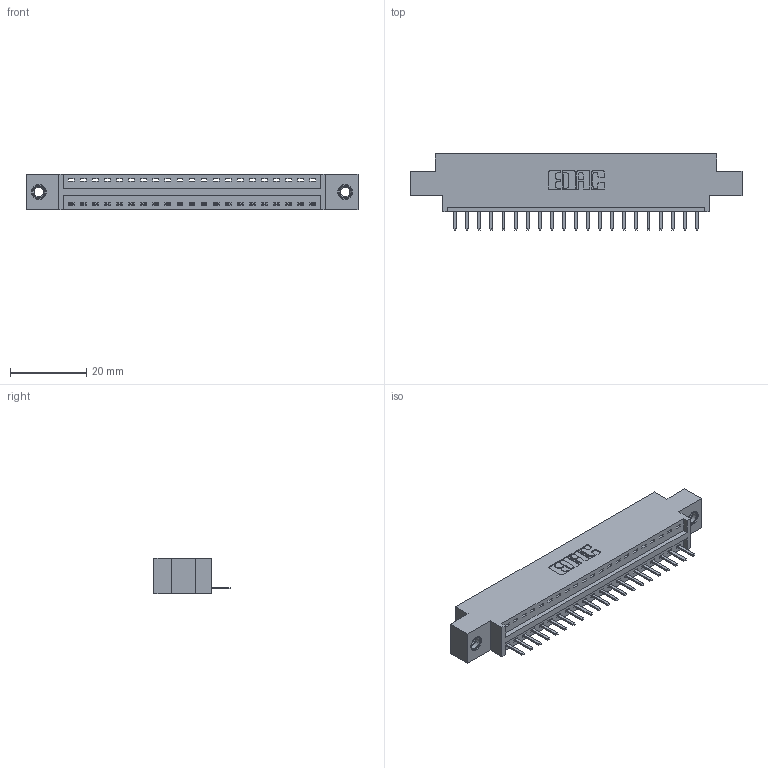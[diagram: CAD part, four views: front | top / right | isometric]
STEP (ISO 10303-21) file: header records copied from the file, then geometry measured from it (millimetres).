
FILE_DESCRIPTION (( 'STEP AP203' ), '1' );
FILE_NAME ('396-021-520-607.STEP', '2019-10-27T03:50:43', ( '' ), ( '' ), 'SwSTEP 2.0', 'SolidWorks 2016', '' );
FILE_SCHEMA (( 'CONFIG_CONTROL_DESIGN' ));
Length unit declared in the file: inch
Products named in the file (4): 346 Part_0.170 Offset - 0.156 Dia-TI; 396-021-520-607; 345-292-001_345-293-120; 345-250-001_345-250-005-103
Assembly tree (24 placements, depth 2):
  396-021-520-607
    346 Part_0.170 Offset - 0.156 Dia-TI
    345-292-001_345-293-120  x21
    345-250-001_345-250-005-103  x2
Bounding box: 87.25 x 20.02 x 9.4 mm (x, y, z)
Volume: 7978.4 mm3; surface area: 9738.7 mm2
Topology: 24 solids, 24 shells, 1488 faces, 4341 edges, 2830 vertices
Faces by surface type: plane 994, cylinder 478, cone 12, torus 4
Entity records: 17292 total; most frequent: CARTESIAN_POINT 2966, ORIENTED_EDGE 2902, DIRECTION 2655, EDGE_CURVE 1451, VECTOR 1211, LINE 1211, VERTEX_POINT 960, AXIS2_PLACEMENT_3D 722
